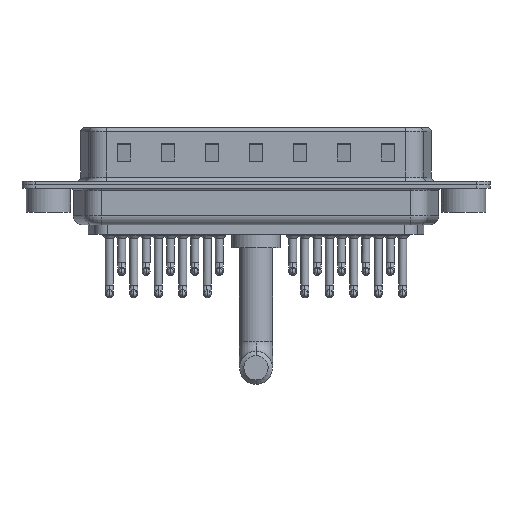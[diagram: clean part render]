
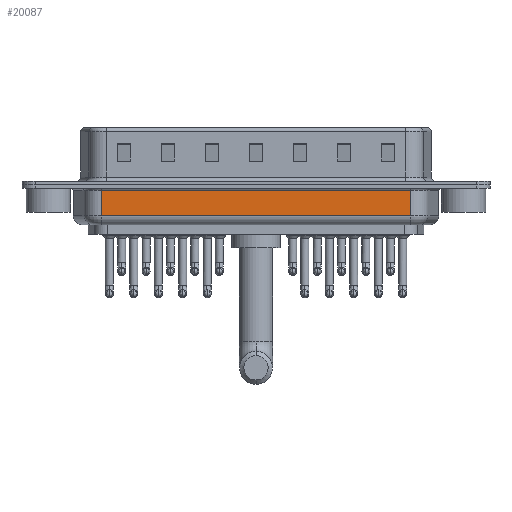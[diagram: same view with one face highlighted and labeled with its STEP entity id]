
A CAD part, front view. The second image highlights one B-rep face of the part: STEP entity #20087.
In plain terms, the highlighted planar face has unit normal (0, -1, 0).
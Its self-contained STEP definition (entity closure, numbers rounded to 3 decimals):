
#65 = VECTOR ( 'NONE', #11291, 1000. ) ;
#125 = EDGE_CURVE ( 'NONE', #388, #25199, #18728, .T. ) ;
#388 = VERTEX_POINT ( 'NONE', #15309 ) ;
#567 = AXIS2_PLACEMENT_3D ( 'NONE', #11115, #12825, #6794 ) ;
#2871 = ORIENTED_EDGE ( 'NONE', *, *, #12822, .T. ) ;
#4431 = DIRECTION ( 'NONE',  ( 0., 0., 1. ) ) ;
#5380 = LINE ( 'NONE', #19665, #65 ) ;
#5927 = VERTEX_POINT ( 'NONE', #12296 ) ;
#5990 = EDGE_CURVE ( 'NONE', #25199, #5927, #8500, .T. ) ;
#6794 = DIRECTION ( 'NONE',  ( 0., 0., 1. ) ) ;
#6898 = EDGE_LOOP ( 'NONE', ( #11839, #12478, #9930, #2871 ) ) ;
#7428 = VECTOR ( 'NONE', #16498, 1000. ) ;
#7785 = EDGE_CURVE ( 'NONE', #388, #21569, #24349, .T. ) ;
#7857 = VECTOR ( 'NONE', #4431, 1000. ) ;
#8500 = LINE ( 'NONE', #22366, #7428 ) ;
#9930 = ORIENTED_EDGE ( 'NONE', *, *, #5990, .T. ) ;
#10764 = VECTOR ( 'NONE', #24466, 1000. ) ;
#11115 = CARTESIAN_POINT ( 'NONE',  ( 6.006, -5.35, -4.5 ) ) ;
#11291 = DIRECTION ( 'NONE',  ( -1., 0., 0. ) ) ;
#11839 = ORIENTED_EDGE ( 'NONE', *, *, #7785, .F. ) ;
#12296 = CARTESIAN_POINT ( 'NONE',  ( 41.044, -5.35, -0.65 ) ) ;
#12478 = ORIENTED_EDGE ( 'NONE', *, *, #125, .T. ) ;
#12822 = EDGE_CURVE ( 'NONE', #5927, #21569, #5380, .T. ) ;
#12825 = DIRECTION ( 'NONE',  ( 0., 1., 0. ) ) ;
#13243 = CARTESIAN_POINT ( 'NONE',  ( 41.044, -5.35, -3.5 ) ) ;
#14285 = CARTESIAN_POINT ( 'NONE',  ( 6.006, -5.35, -4.5 ) ) ;
#15191 = FACE_OUTER_BOUND ( 'NONE', #6898, .T. ) ;
#15309 = CARTESIAN_POINT ( 'NONE',  ( 6.006, -5.35, -3.5 ) ) ;
#16498 = DIRECTION ( 'NONE',  ( 0., 0., 1. ) ) ;
#16501 = CARTESIAN_POINT ( 'NONE',  ( 6.006, -5.35, -3.5 ) ) ;
#18728 = LINE ( 'NONE', #16501, #10764 ) ;
#19665 = CARTESIAN_POINT ( 'NONE',  ( 6.006, -5.35, -0.65 ) ) ;
#20087 = ADVANCED_FACE ( 'NONE', ( #15191 ), #25004, .F. ) ;
#21569 = VERTEX_POINT ( 'NONE', #24444 ) ;
#22366 = CARTESIAN_POINT ( 'NONE',  ( 41.044, -5.35, -4.5 ) ) ;
#24349 = LINE ( 'NONE', #14285, #7857 ) ;
#24444 = CARTESIAN_POINT ( 'NONE',  ( 6.006, -5.35, -0.65 ) ) ;
#24466 = DIRECTION ( 'NONE',  ( 1., 0., 0. ) ) ;
#25004 = PLANE ( 'NONE',  #567 ) ;
#25199 = VERTEX_POINT ( 'NONE', #13243 ) ;
